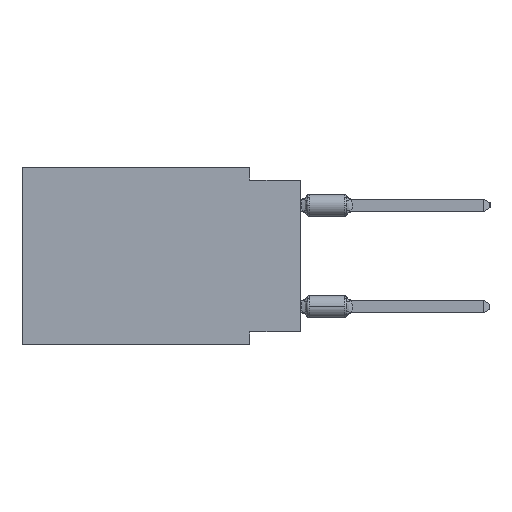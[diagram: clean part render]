
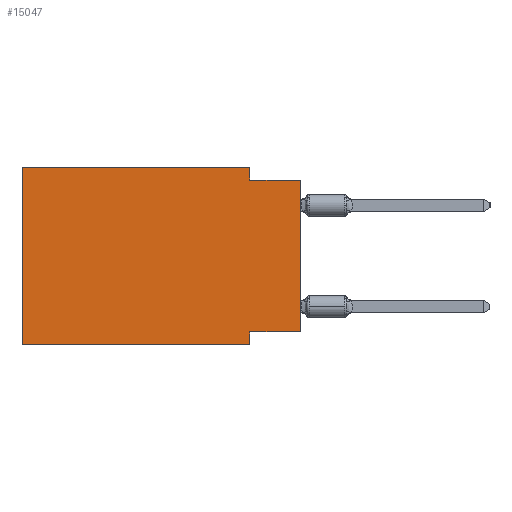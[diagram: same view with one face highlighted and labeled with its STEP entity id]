
A CAD part, left-side view. The second image highlights one B-rep face of the part: STEP entity #15047.
In plain terms, the highlighted planar face has unit normal (-1, 0, 0).
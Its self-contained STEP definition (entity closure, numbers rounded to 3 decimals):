
#918 = VERTEX_POINT ( 'NONE', #43522 ) ;
#963 = CARTESIAN_POINT ( 'NONE',  ( 0., 0., -0.635 ) ) ;
#1322 = DIRECTION ( 'NONE',  ( 0., 0., -1. ) ) ;
#1652 = LINE ( 'NONE', #26267, #17361 ) ;
#3308 = ORIENTED_EDGE ( 'NONE', *, *, #15820, .T. ) ;
#3657 = VECTOR ( 'NONE', #27753, 1000. ) ;
#4346 = VECTOR ( 'NONE', #45165, 1000. ) ;
#4631 = CARTESIAN_POINT ( 'NONE',  ( 0., 13.97, 0. ) ) ;
#4950 = DIRECTION ( 'NONE',  ( 0., 0., -1. ) ) ;
#5365 = VERTEX_POINT ( 'NONE', #23847 ) ;
#5776 = ORIENTED_EDGE ( 'NONE', *, *, #25212, .F. ) ;
#6395 = CARTESIAN_POINT ( 'NONE',  ( 0., 13.97, -8.89 ) ) ;
#8446 = VERTEX_POINT ( 'NONE', #38141 ) ;
#9230 = VECTOR ( 'NONE', #18484, 1000. ) ;
#9730 = LINE ( 'NONE', #6395, #19310 ) ;
#10429 = ORIENTED_EDGE ( 'NONE', *, *, #18975, .F. ) ;
#11187 = EDGE_LOOP ( 'NONE', ( #3308, #5776, #30958, #28379, #31330, #42130, #10429, #34853 ) ) ;
#12951 = EDGE_CURVE ( 'NONE', #918, #5365, #25342, .T. ) ;
#13483 = EDGE_CURVE ( 'NONE', #20802, #31364, #25520, .T. ) ;
#14127 = VECTOR ( 'NONE', #32201, 1000. ) ;
#14224 = VERTEX_POINT ( 'NONE', #24943 ) ;
#15047 = ADVANCED_FACE ( 'NONE', ( #15549 ), #44151, .F. ) ;
#15549 = FACE_OUTER_BOUND ( 'NONE', #11187, .T. ) ;
#15820 = EDGE_CURVE ( 'NONE', #918, #14224, #46642, .T. ) ;
#17361 = VECTOR ( 'NONE', #4950, 1000. ) ;
#17787 = VERTEX_POINT ( 'NONE', #45176 ) ;
#18484 = DIRECTION ( 'NONE',  ( 0., -1., 0. ) ) ;
#18975 = EDGE_CURVE ( 'NONE', #5365, #8446, #1652, .T. ) ;
#19310 = VECTOR ( 'NONE', #25074, 1000. ) ;
#20802 = VERTEX_POINT ( 'NONE', #44334 ) ;
#21784 = EDGE_CURVE ( 'NONE', #39325, #20802, #23864, .T. ) ;
#22628 = DIRECTION ( 'NONE',  ( 1., 0., 0. ) ) ;
#23847 = CARTESIAN_POINT ( 'NONE',  ( 0., 2.54, -8.255 ) ) ;
#23864 = LINE ( 'NONE', #31436, #4346 ) ;
#24934 = VECTOR ( 'NONE', #38214, 1000. ) ;
#24943 = CARTESIAN_POINT ( 'NONE',  ( 0., 0., -0.635 ) ) ;
#25074 = DIRECTION ( 'NONE',  ( 0., -1., 0. ) ) ;
#25212 = EDGE_CURVE ( 'NONE', #17787, #14224, #44254, .T. ) ;
#25342 = LINE ( 'NONE', #31976, #14127 ) ;
#25520 = LINE ( 'NONE', #32847, #28425 ) ;
#26267 = CARTESIAN_POINT ( 'NONE',  ( 0., 2.54, -8.89 ) ) ;
#27753 = DIRECTION ( 'NONE',  ( 0., 0., 1. ) ) ;
#28379 = ORIENTED_EDGE ( 'NONE', *, *, #13483, .F. ) ;
#28425 = VECTOR ( 'NONE', #40636, 1000. ) ;
#30805 = AXIS2_PLACEMENT_3D ( 'NONE', #4631, #22628, #1322 ) ;
#30893 = LINE ( 'NONE', #45787, #24934 ) ;
#30938 = EDGE_CURVE ( 'NONE', #31364, #17787, #30893, .T. ) ;
#30958 = ORIENTED_EDGE ( 'NONE', *, *, #30938, .F. ) ;
#31330 = ORIENTED_EDGE ( 'NONE', *, *, #21784, .F. ) ;
#31364 = VERTEX_POINT ( 'NONE', #40996 ) ;
#31436 = CARTESIAN_POINT ( 'NONE',  ( 0., 13.97, 0. ) ) ;
#31976 = CARTESIAN_POINT ( 'NONE',  ( 0., 0., -8.255 ) ) ;
#32201 = DIRECTION ( 'NONE',  ( 0., 1., 0. ) ) ;
#32847 = CARTESIAN_POINT ( 'NONE',  ( 0., 13.97, 0. ) ) ;
#34853 = ORIENTED_EDGE ( 'NONE', *, *, #12951, .F. ) ;
#35531 = CARTESIAN_POINT ( 'NONE',  ( 0., 0., 0. ) ) ;
#37746 = CARTESIAN_POINT ( 'NONE',  ( 0., 13.97, -8.89 ) ) ;
#38141 = CARTESIAN_POINT ( 'NONE',  ( 0., 2.54, -8.89 ) ) ;
#38214 = DIRECTION ( 'NONE',  ( 0., 0., -1. ) ) ;
#39325 = VERTEX_POINT ( 'NONE', #37746 ) ;
#40636 = DIRECTION ( 'NONE',  ( 0., -1., 0. ) ) ;
#40996 = CARTESIAN_POINT ( 'NONE',  ( 0., 2.54, 0. ) ) ;
#42130 = ORIENTED_EDGE ( 'NONE', *, *, #44487, .T. ) ;
#43522 = CARTESIAN_POINT ( 'NONE',  ( 0., 0., -8.255 ) ) ;
#44151 = PLANE ( 'NONE',  #30805 ) ;
#44254 = LINE ( 'NONE', #963, #9230 ) ;
#44334 = CARTESIAN_POINT ( 'NONE',  ( 0., 13.97, 0. ) ) ;
#44487 = EDGE_CURVE ( 'NONE', #39325, #8446, #9730, .T. ) ;
#45165 = DIRECTION ( 'NONE',  ( 0., 0., 1. ) ) ;
#45176 = CARTESIAN_POINT ( 'NONE',  ( 0., 2.54, -0.635 ) ) ;
#45787 = CARTESIAN_POINT ( 'NONE',  ( 0., 2.54, 0. ) ) ;
#46642 = LINE ( 'NONE', #35531, #3657 ) ;
